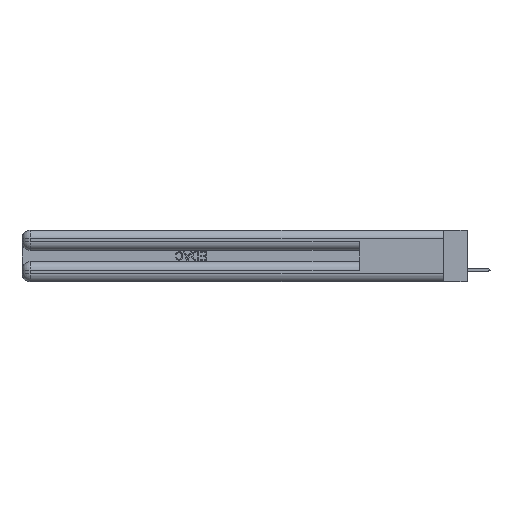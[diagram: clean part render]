
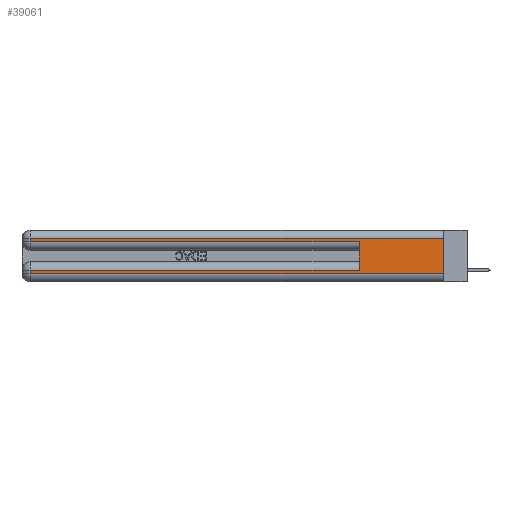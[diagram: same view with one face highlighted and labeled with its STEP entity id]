
A CAD part, left-side view. The second image highlights one B-rep face of the part: STEP entity #39061.
In plain terms, the highlighted planar face has unit normal (-1, 0, 0).
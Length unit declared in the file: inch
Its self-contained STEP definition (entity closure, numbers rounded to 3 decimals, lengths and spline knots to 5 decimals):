
#1371 = CARTESIAN_POINT ( 'NONE',  ( 0., 2.94, 0.085 ) ) ;
#1502 = CARTESIAN_POINT ( 'NONE',  ( 0., 0., 0.37 ) ) ;
#2129 = CARTESIAN_POINT ( 'NONE',  ( 0., 0., 0.085 ) ) ;
#2611 = VERTEX_POINT ( 'NONE', #18770 ) ;
#3508 = VERTEX_POINT ( 'NONE', #12997 ) ;
#4383 = CARTESIAN_POINT ( 'NONE',  ( 0., 0., 0.31 ) ) ;
#5141 = CARTESIAN_POINT ( 'NONE',  ( 0., 2.94, 0.31 ) ) ;
#5648 = DIRECTION ( 'NONE',  ( 0., 0., -1. ) ) ;
#8493 = CARTESIAN_POINT ( 'NONE',  ( 0., 2.94, 0.06 ) ) ;
#8655 = LINE ( 'NONE', #4383, #37177 ) ;
#10011 = CARTESIAN_POINT ( 'NONE',  ( 0., 2.94, 0.37 ) ) ;
#10274 = LINE ( 'NONE', #34788, #52397 ) ;
#10859 = DIRECTION ( 'NONE',  ( 0., 0., -1. ) ) ;
#12997 = CARTESIAN_POINT ( 'NONE',  ( 0., 2.94, 0.285 ) ) ;
#13328 = DIRECTION ( 'NONE',  ( 0., -1., 0. ) ) ;
#14342 = CARTESIAN_POINT ( 'NONE',  ( 0., 0.6, 0.285 ) ) ;
#14879 = ORIENTED_EDGE ( 'NONE', *, *, #39409, .T. ) ;
#15875 = VECTOR ( 'NONE', #18470, 39.37008 ) ;
#17809 = LINE ( 'NONE', #2129, #15875 ) ;
#18470 = DIRECTION ( 'NONE',  ( 0., 1., 0. ) ) ;
#18770 = CARTESIAN_POINT ( 'NONE',  ( 0., 0.6, 0.085 ) ) ;
#21294 = DIRECTION ( 'NONE',  ( 0., -1., 0. ) ) ;
#21348 = ORIENTED_EDGE ( 'NONE', *, *, #42288, .T. ) ;
#21852 = PLANE ( 'NONE',  #52193 ) ;
#22043 = DIRECTION ( 'NONE',  ( 0., 0., -1. ) ) ;
#24361 = EDGE_CURVE ( 'NONE', #2611, #52932, #17809, .T. ) ;
#25305 = VERTEX_POINT ( 'NONE', #41819 ) ;
#25448 = LINE ( 'NONE', #27215, #47472 ) ;
#25991 = VERTEX_POINT ( 'NONE', #5141 ) ;
#26259 = ORIENTED_EDGE ( 'NONE', *, *, #24361, .T. ) ;
#26343 = ORIENTED_EDGE ( 'NONE', *, *, #28992, .F. ) ;
#27215 = CARTESIAN_POINT ( 'NONE',  ( 0., 0., 0.37 ) ) ;
#28992 = EDGE_CURVE ( 'NONE', #2611, #38853, #10274, .T. ) ;
#29344 = VERTEX_POINT ( 'NONE', #8493 ) ;
#30798 = DIRECTION ( 'NONE',  ( 0., 0., 1. ) ) ;
#32676 = VERTEX_POINT ( 'NONE', #39222 ) ;
#32965 = EDGE_CURVE ( 'NONE', #29344, #32676, #38764, .T. ) ;
#34788 = CARTESIAN_POINT ( 'NONE',  ( 0., 0.6, 0.145 ) ) ;
#34803 = DIRECTION ( 'NONE',  ( 1., 0., 0. ) ) ;
#34898 = VECTOR ( 'NONE', #13328, 39.37008 ) ;
#34964 = LINE ( 'NONE', #41960, #34898 ) ;
#35264 = EDGE_CURVE ( 'NONE', #52932, #29344, #45694, .T. ) ;
#37177 = VECTOR ( 'NONE', #37470, 39.37008 ) ;
#37363 = EDGE_CURVE ( 'NONE', #25991, #3508, #53071, .T. ) ;
#37470 = DIRECTION ( 'NONE',  ( 0., 1., 0. ) ) ;
#38764 = LINE ( 'NONE', #41207, #40076 ) ;
#38853 = VERTEX_POINT ( 'NONE', #14342 ) ;
#39061 = ADVANCED_FACE ( 'NONE', ( #49583 ), #21852, .F. ) ;
#39222 = CARTESIAN_POINT ( 'NONE',  ( 0., 0., 0.06 ) ) ;
#39409 = EDGE_CURVE ( 'NONE', #25305, #25991, #8655, .T. ) ;
#39955 = ORIENTED_EDGE ( 'NONE', *, *, #37363, .T. ) ;
#40076 = VECTOR ( 'NONE', #21294, 39.37008 ) ;
#41207 = CARTESIAN_POINT ( 'NONE',  ( 0., 0., 0.06 ) ) ;
#41288 = EDGE_LOOP ( 'NONE', ( #47655, #14879, #39955, #21348, #26343, #26259, #46328, #52009 ) ) ;
#41819 = CARTESIAN_POINT ( 'NONE',  ( 0., 0., 0.31 ) ) ;
#41960 = CARTESIAN_POINT ( 'NONE',  ( 0., 0., 0.285 ) ) ;
#42288 = EDGE_CURVE ( 'NONE', #3508, #38853, #34964, .T. ) ;
#44069 = DIRECTION ( 'NONE',  ( 0., 0., -1. ) ) ;
#45694 = LINE ( 'NONE', #10011, #52137 ) ;
#46328 = ORIENTED_EDGE ( 'NONE', *, *, #35264, .T. ) ;
#46559 = VECTOR ( 'NONE', #10859, 39.37008 ) ;
#47422 = EDGE_CURVE ( 'NONE', #25305, #32676, #25448, .T. ) ;
#47472 = VECTOR ( 'NONE', #44069, 39.37008 ) ;
#47655 = ORIENTED_EDGE ( 'NONE', *, *, #47422, .F. ) ;
#47872 = CARTESIAN_POINT ( 'NONE',  ( 0., 2.94, 0.37 ) ) ;
#49583 = FACE_OUTER_BOUND ( 'NONE', #41288, .T. ) ;
#52009 = ORIENTED_EDGE ( 'NONE', *, *, #32965, .T. ) ;
#52137 = VECTOR ( 'NONE', #22043, 39.37008 ) ;
#52193 = AXIS2_PLACEMENT_3D ( 'NONE', #1502, #34803, #5648 ) ;
#52397 = VECTOR ( 'NONE', #30798, 39.37008 ) ;
#52932 = VERTEX_POINT ( 'NONE', #1371 ) ;
#53071 = LINE ( 'NONE', #47872, #46559 ) ;
